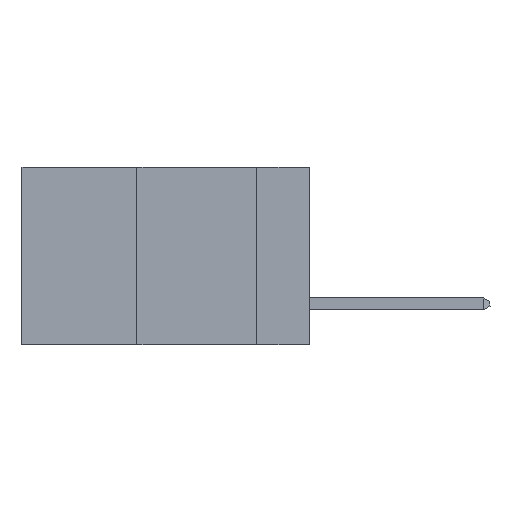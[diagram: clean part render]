
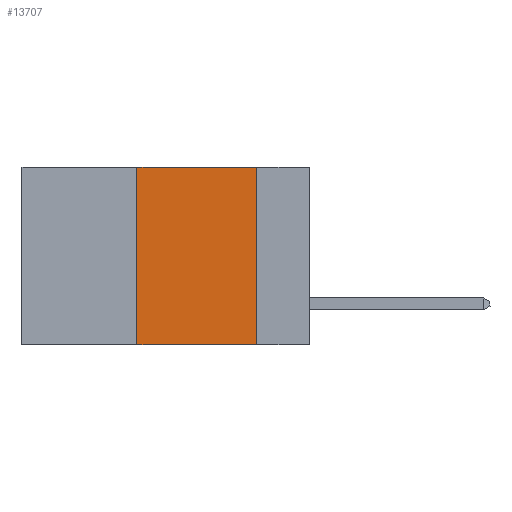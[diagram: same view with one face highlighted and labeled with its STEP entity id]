
A CAD part, left-side view. The second image highlights one B-rep face of the part: STEP entity #13707.
In plain terms, the highlighted planar face has unit normal (-1, 0, 0).
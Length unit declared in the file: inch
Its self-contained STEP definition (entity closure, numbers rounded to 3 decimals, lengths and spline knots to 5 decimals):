
#535 = ORIENTED_EDGE ( 'NONE', *, *, #33612, .F. ) ;
#755 = CARTESIAN_POINT ( 'NONE',  ( 0., 0.36, 0. ) ) ;
#1125 = VECTOR ( 'NONE', #5179, 39.37008 ) ;
#3051 = FACE_OUTER_BOUND ( 'NONE', #29986, .T. ) ;
#3503 = DIRECTION ( 'NONE',  ( 0., 0., 1. ) ) ;
#4321 = LINE ( 'NONE', #29016, #11891 ) ;
#4842 = ORIENTED_EDGE ( 'NONE', *, *, #24226, .F. ) ;
#5179 = DIRECTION ( 'NONE',  ( 0., -1., 0. ) ) ;
#5254 = CARTESIAN_POINT ( 'NONE',  ( 0., 0.6, 0. ) ) ;
#6637 = CARTESIAN_POINT ( 'NONE',  ( 0., 0.11, -0.37 ) ) ;
#7718 = CARTESIAN_POINT ( 'NONE',  ( 0., 0.11, 0. ) ) ;
#8032 = CARTESIAN_POINT ( 'NONE',  ( 0., 0.6, -0.37 ) ) ;
#8114 = DIRECTION ( 'NONE',  ( 1., 0., 0. ) ) ;
#9854 = LINE ( 'NONE', #15214, #31527 ) ;
#9873 = ORIENTED_EDGE ( 'NONE', *, *, #30634, .F. ) ;
#10979 = CARTESIAN_POINT ( 'NONE',  ( 0., 0.11, 0. ) ) ;
#11891 = VECTOR ( 'NONE', #3503, 39.37008 ) ;
#13204 = VERTEX_POINT ( 'NONE', #6637 ) ;
#13707 = ADVANCED_FACE ( 'NONE', ( #3051 ), #22246, .F. ) ;
#15214 = CARTESIAN_POINT ( 'NONE',  ( 0., 0.6, 0. ) ) ;
#15285 = VERTEX_POINT ( 'NONE', #31755 ) ;
#21045 = VERTEX_POINT ( 'NONE', #7718 ) ;
#22246 = PLANE ( 'NONE',  #25669 ) ;
#23055 = EDGE_CURVE ( 'NONE', #15285, #13204, #23727, .T. ) ;
#23727 = LINE ( 'NONE', #8032, #1125 ) ;
#24226 = EDGE_CURVE ( 'NONE', #21045, #13204, #26284, .T. ) ;
#24504 = VERTEX_POINT ( 'NONE', #755 ) ;
#25669 = AXIS2_PLACEMENT_3D ( 'NONE', #5254, #8114, #27932 ) ;
#26284 = LINE ( 'NONE', #10979, #34677 ) ;
#27028 = ORIENTED_EDGE ( 'NONE', *, *, #23055, .T. ) ;
#27932 = DIRECTION ( 'NONE',  ( 0., 0., -1. ) ) ;
#29016 = CARTESIAN_POINT ( 'NONE',  ( 0., 0.36, 0. ) ) ;
#29309 = DIRECTION ( 'NONE',  ( 0., -1., 0. ) ) ;
#29986 = EDGE_LOOP ( 'NONE', ( #4842, #535, #9873, #27028 ) ) ;
#30634 = EDGE_CURVE ( 'NONE', #15285, #24504, #4321, .T. ) ;
#30746 = DIRECTION ( 'NONE',  ( 0., 0., -1. ) ) ;
#31527 = VECTOR ( 'NONE', #29309, 39.37008 ) ;
#31755 = CARTESIAN_POINT ( 'NONE',  ( 0., 0.36, -0.37 ) ) ;
#33612 = EDGE_CURVE ( 'NONE', #24504, #21045, #9854, .T. ) ;
#34677 = VECTOR ( 'NONE', #30746, 39.37008 ) ;
